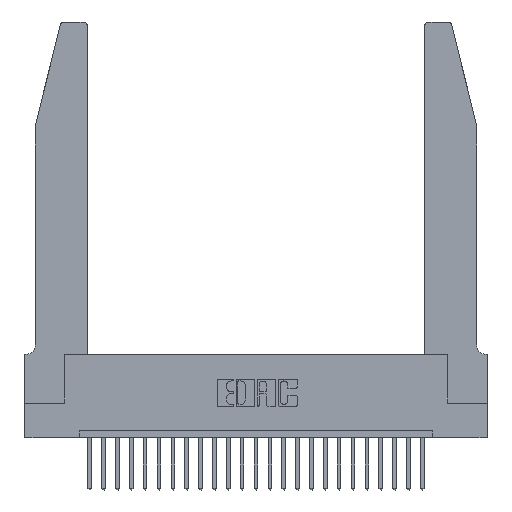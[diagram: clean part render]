
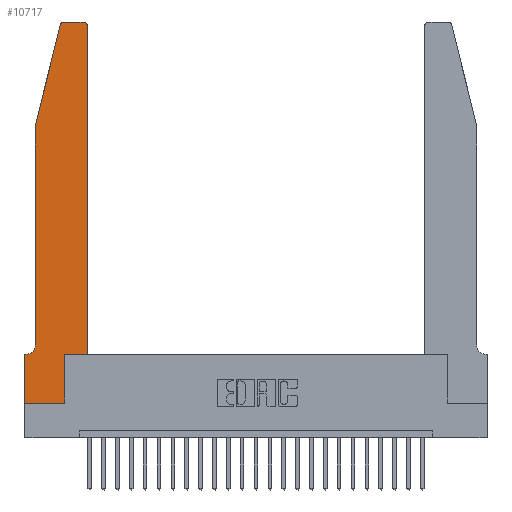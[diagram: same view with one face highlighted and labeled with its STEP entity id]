
A CAD part, top view. The second image highlights one B-rep face of the part: STEP entity #10717.
In plain terms, the highlighted planar face has unit normal (0, 0, 1).
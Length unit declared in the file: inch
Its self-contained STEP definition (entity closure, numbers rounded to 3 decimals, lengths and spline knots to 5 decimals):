
#12 = ORIENTED_EDGE ( 'NONE', *, *, #24867, .T. ) ;
#572 = EDGE_CURVE ( 'NONE', #6477, #2951, #11177, .T. ) ;
#752 = DIRECTION ( 'NONE',  ( 0., 0., 1. ) ) ;
#863 = VECTOR ( 'NONE', #10807, 39.37008 ) ;
#1270 = LINE ( 'NONE', #7422, #9683 ) ;
#1599 = ORIENTED_EDGE ( 'NONE', *, *, #9069, .T. ) ;
#1935 = LINE ( 'NONE', #4914, #20652 ) ;
#2385 = LINE ( 'NONE', #25494, #4881 ) ;
#2491 = DIRECTION ( 'NONE',  ( 1., 0., 0. ) ) ;
#2582 = DIRECTION ( 'NONE',  ( 1., 0., 0. ) ) ;
#2608 = VERTEX_POINT ( 'NONE', #20278 ) ;
#2760 = VERTEX_POINT ( 'NONE', #4765 ) ;
#2930 = CARTESIAN_POINT ( 'NONE',  ( 0.0755, 0.42, 0.37 ) ) ;
#2951 = VERTEX_POINT ( 'NONE', #9724 ) ;
#2959 = CARTESIAN_POINT ( 'NONE',  ( 0.25487, 2.72718, 0.37 ) ) ;
#3540 = EDGE_LOOP ( 'NONE', ( #12404, #16977, #18382, #22992, #10560, #1599, #4869, #12, #13395, #16158, #5838, #9578 ) ) ;
#3909 = CIRCLE ( 'NONE', #10551, 0.03 ) ;
#4082 = EDGE_CURVE ( 'NONE', #25353, #13310, #5409, .T. ) ;
#4481 = LINE ( 'NONE', #17243, #11664 ) ;
#4765 = CARTESIAN_POINT ( 'NONE',  ( 0., 0.35, 0.37 ) ) ;
#4778 = CARTESIAN_POINT ( 'NONE',  ( 0.284, 2.75, 0.37 ) ) ;
#4792 = EDGE_CURVE ( 'NONE', #5122, #6477, #1935, .T. ) ;
#4837 = LINE ( 'NONE', #14960, #7631 ) ;
#4869 = ORIENTED_EDGE ( 'NONE', *, *, #15128, .T. ) ;
#4881 = VECTOR ( 'NONE', #23673, 39.37008 ) ;
#4914 = CARTESIAN_POINT ( 'NONE',  ( 0.4505, 0.35, 0.37 ) ) ;
#5122 = VERTEX_POINT ( 'NONE', #22062 ) ;
#5409 = LINE ( 'NONE', #11210, #19120 ) ;
#5767 = AXIS2_PLACEMENT_3D ( 'NONE', #14608, #24494, #2582 ) ;
#5838 = ORIENTED_EDGE ( 'NONE', *, *, #4792, .T. ) ;
#6260 = VECTOR ( 'NONE', #14353, 39.37008 ) ;
#6477 = VERTEX_POINT ( 'NONE', #13576 ) ;
#7399 = LINE ( 'NONE', #20609, #863 ) ;
#7422 = CARTESIAN_POINT ( 'NONE',  ( 0., 0., 0.37 ) ) ;
#7631 = VECTOR ( 'NONE', #11118, 39.37008 ) ;
#7878 = AXIS2_PLACEMENT_3D ( 'NONE', #10524, #18387, #20736 ) ;
#7890 = CARTESIAN_POINT ( 'NONE',  ( 0.2865, 0.35, 0.37 ) ) ;
#8209 = CARTESIAN_POINT ( 'NONE',  ( 0.0755, 2., 0.37 ) ) ;
#8517 = PLANE ( 'NONE',  #5767 ) ;
#8724 = CARTESIAN_POINT ( 'NONE',  ( 0., 0., 0.37 ) ) ;
#9069 = EDGE_CURVE ( 'NONE', #20310, #2760, #10295, .T. ) ;
#9578 = ORIENTED_EDGE ( 'NONE', *, *, #572, .T. ) ;
#9683 = VECTOR ( 'NONE', #15368, 39.37008 ) ;
#9724 = CARTESIAN_POINT ( 'NONE',  ( 0.4205, 2.75, 0.37 ) ) ;
#10295 = LINE ( 'NONE', #20461, #6260 ) ;
#10524 = CARTESIAN_POINT ( 'NONE',  ( 0.0055, 0.42, 0.37 ) ) ;
#10551 = AXIS2_PLACEMENT_3D ( 'NONE', #15908, #752, #2491 ) ;
#10560 = ORIENTED_EDGE ( 'NONE', *, *, #16885, .T. ) ;
#10717 = ADVANCED_FACE ( 'NONE', ( #21764 ), #8517, .T. ) ;
#10807 = DIRECTION ( 'NONE',  ( 0., -1., 0. ) ) ;
#10947 = DIRECTION ( 'NONE',  ( -0.239, -0.971, 0. ) ) ;
#11118 = DIRECTION ( 'NONE',  ( 0., 1., 0. ) ) ;
#11177 = CIRCLE ( 'NONE', #18760, 0.03 ) ;
#11210 = CARTESIAN_POINT ( 'NONE',  ( 0.0755, 2., 0.37 ) ) ;
#11664 = VECTOR ( 'NONE', #13251, 39.37008 ) ;
#11873 = DIRECTION ( 'NONE',  ( 1., 0., 0. ) ) ;
#12292 = CIRCLE ( 'NONE', #7878, 0.07 ) ;
#12404 = ORIENTED_EDGE ( 'NONE', *, *, #15627, .T. ) ;
#13251 = DIRECTION ( 'NONE',  ( 1., 0., 0. ) ) ;
#13310 = VERTEX_POINT ( 'NONE', #8209 ) ;
#13395 = ORIENTED_EDGE ( 'NONE', *, *, #16588, .T. ) ;
#13576 = CARTESIAN_POINT ( 'NONE',  ( 0.4505, 2.72, 0.37 ) ) ;
#14353 = DIRECTION ( 'NONE',  ( -1., 0., 0. ) ) ;
#14608 = CARTESIAN_POINT ( 'NONE',  ( 0., 0.35, 0.37 ) ) ;
#14960 = CARTESIAN_POINT ( 'NONE',  ( 0.2865, 0.35, 0.37 ) ) ;
#15128 = EDGE_CURVE ( 'NONE', #2760, #2608, #20840, .T. ) ;
#15368 = DIRECTION ( 'NONE',  ( 1., 0., 0. ) ) ;
#15510 = VECTOR ( 'NONE', #25618, 39.37008 ) ;
#15627 = EDGE_CURVE ( 'NONE', #2951, #25741, #2385, .T. ) ;
#15908 = CARTESIAN_POINT ( 'NONE',  ( 0.284, 2.72, 0.37 ) ) ;
#16036 = EDGE_CURVE ( 'NONE', #25741, #25353, #3909, .T. ) ;
#16062 = VERTEX_POINT ( 'NONE', #19069 ) ;
#16158 = ORIENTED_EDGE ( 'NONE', *, *, #25443, .T. ) ;
#16588 = EDGE_CURVE ( 'NONE', #16062, #21597, #4837, .T. ) ;
#16885 = EDGE_CURVE ( 'NONE', #22014, #20310, #12292, .T. ) ;
#16977 = ORIENTED_EDGE ( 'NONE', *, *, #16036, .T. ) ;
#17243 = CARTESIAN_POINT ( 'NONE',  ( 0.4505, 0.35, 0.37 ) ) ;
#18382 = ORIENTED_EDGE ( 'NONE', *, *, #4082, .T. ) ;
#18387 = DIRECTION ( 'NONE',  ( 0., 0., -1. ) ) ;
#18760 = AXIS2_PLACEMENT_3D ( 'NONE', #19444, #25568, #11873 ) ;
#18954 = DIRECTION ( 'NONE',  ( 0., 1., 0. ) ) ;
#19069 = CARTESIAN_POINT ( 'NONE',  ( 0.2865, 0., 0.37 ) ) ;
#19120 = VECTOR ( 'NONE', #10947, 39.37008 ) ;
#19444 = CARTESIAN_POINT ( 'NONE',  ( 0.4205, 2.72, 0.37 ) ) ;
#19773 = EDGE_CURVE ( 'NONE', #13310, #22014, #7399, .T. ) ;
#20278 = CARTESIAN_POINT ( 'NONE',  ( 0., 0., 0.37 ) ) ;
#20310 = VERTEX_POINT ( 'NONE', #21594 ) ;
#20461 = CARTESIAN_POINT ( 'NONE',  ( 0.0755, 0.35, 0.37 ) ) ;
#20609 = CARTESIAN_POINT ( 'NONE',  ( 0.0755, 2., 0.37 ) ) ;
#20652 = VECTOR ( 'NONE', #18954, 39.37008 ) ;
#20736 = DIRECTION ( 'NONE',  ( -1., 0., 0. ) ) ;
#20840 = LINE ( 'NONE', #8724, #15510 ) ;
#21594 = CARTESIAN_POINT ( 'NONE',  ( 0.0055, 0.35, 0.37 ) ) ;
#21597 = VERTEX_POINT ( 'NONE', #7890 ) ;
#21764 = FACE_OUTER_BOUND ( 'NONE', #3540, .T. ) ;
#22014 = VERTEX_POINT ( 'NONE', #2930 ) ;
#22062 = CARTESIAN_POINT ( 'NONE',  ( 0.4505, 0.35, 0.37 ) ) ;
#22992 = ORIENTED_EDGE ( 'NONE', *, *, #19773, .T. ) ;
#23673 = DIRECTION ( 'NONE',  ( -1., 0., 0. ) ) ;
#24494 = DIRECTION ( 'NONE',  ( 0., 0., 1. ) ) ;
#24867 = EDGE_CURVE ( 'NONE', #2608, #16062, #1270, .T. ) ;
#25353 = VERTEX_POINT ( 'NONE', #2959 ) ;
#25443 = EDGE_CURVE ( 'NONE', #21597, #5122, #4481, .T. ) ;
#25494 = CARTESIAN_POINT ( 'NONE',  ( 0.2605, 2.75, 0.37 ) ) ;
#25568 = DIRECTION ( 'NONE',  ( 0., 0., 1. ) ) ;
#25618 = DIRECTION ( 'NONE',  ( 0., -1., 0. ) ) ;
#25741 = VERTEX_POINT ( 'NONE', #4778 ) ;
